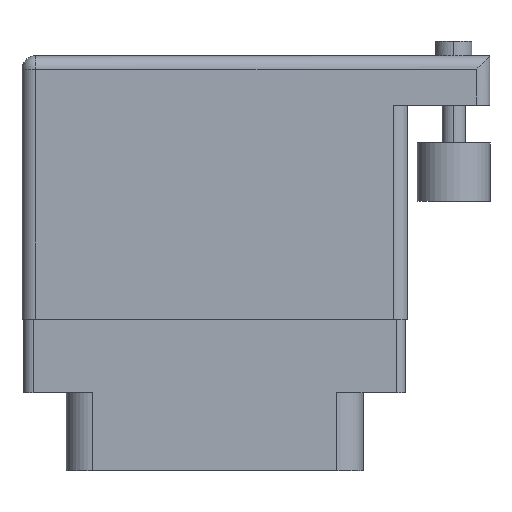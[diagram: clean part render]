
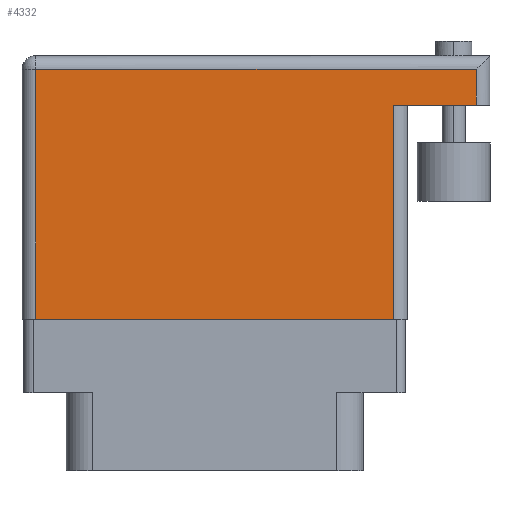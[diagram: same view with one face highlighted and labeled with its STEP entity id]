
A CAD part, front view. The second image highlights one B-rep face of the part: STEP entity #4332.
In plain terms, the highlighted face is planar.
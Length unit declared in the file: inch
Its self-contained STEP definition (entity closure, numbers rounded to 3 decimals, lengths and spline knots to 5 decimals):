
#379 = EDGE_CURVE ( 'NONE', #4389, #19625, #25853, .T. ) ;
#608 = EDGE_CURVE ( 'NONE', #2554, #6173, #16912, .T. ) ;
#660 = VECTOR ( 'NONE', #26076, 39.37008 ) ;
#966 = CARTESIAN_POINT ( 'NONE',  ( 1.278, 0.736, 0. ) ) ;
#1484 = VECTOR ( 'NONE', #26105, 39.37008 ) ;
#1532 = EDGE_LOOP ( 'NONE', ( #11667, #21692, #9767, #13888, #3674, #26341 ) ) ;
#2554 = VERTEX_POINT ( 'NONE', #25929 ) ;
#2714 = FACE_OUTER_BOUND ( 'NONE', #1532, .T. ) ;
#3550 = VERTEX_POINT ( 'NONE', #9226 ) ;
#3674 = ORIENTED_EDGE ( 'NONE', *, *, #4164, .T. ) ;
#3923 = DIRECTION ( 'NONE',  ( -1., 0., 0. ) ) ;
#4164 = EDGE_CURVE ( 'NONE', #6173, #3550, #26039, .T. ) ;
#4332 = ADVANCED_FACE ( 'NONE', ( #2714 ), #6448, .F. ) ;
#4389 = VERTEX_POINT ( 'NONE', #18974 ) ;
#4541 = CARTESIAN_POINT ( 'NONE',  ( 1.562, 0.859, 0. ) ) ;
#6173 = VERTEX_POINT ( 'NONE', #4541 ) ;
#6448 = PLANE ( 'NONE',  #23777 ) ;
#6714 = CARTESIAN_POINT ( 'NONE',  ( 0., 0.906, 0. ) ) ;
#6753 = LINE ( 'NONE', #9155, #11820 ) ;
#6914 = EDGE_CURVE ( 'NONE', #3550, #4389, #26202, .T. ) ;
#7649 = VERTEX_POINT ( 'NONE', #966 ) ;
#7923 = CARTESIAN_POINT ( 'NONE',  ( 0., 0.859, 0. ) ) ;
#9048 = CARTESIAN_POINT ( 'NONE',  ( 1.562, 0.906, 0. ) ) ;
#9155 = CARTESIAN_POINT ( 'NONE',  ( 1.278, 0.736, 0. ) ) ;
#9226 = CARTESIAN_POINT ( 'NONE',  ( 0.047, 0.859, 0. ) ) ;
#9767 = ORIENTED_EDGE ( 'NONE', *, *, #12261, .F. ) ;
#11430 = VECTOR ( 'NONE', #3923, 39.37008 ) ;
#11667 = ORIENTED_EDGE ( 'NONE', *, *, #379, .T. ) ;
#11820 = VECTOR ( 'NONE', #16752, 39.37008 ) ;
#12261 = EDGE_CURVE ( 'NONE', #2554, #7649, #13103, .T. ) ;
#12764 = VECTOR ( 'NONE', #19320, 39.37008 ) ;
#12830 = DIRECTION ( 'NONE',  ( -1., 0., 0. ) ) ;
#13103 = LINE ( 'NONE', #19375, #13503 ) ;
#13503 = VECTOR ( 'NONE', #24946, 39.37008 ) ;
#13888 = ORIENTED_EDGE ( 'NONE', *, *, #608, .T. ) ;
#13991 = CARTESIAN_POINT ( 'NONE',  ( 0., 0., 0. ) ) ;
#16161 = CARTESIAN_POINT ( 'NONE',  ( 1.278, 0., 0. ) ) ;
#16752 = DIRECTION ( 'NONE',  ( 0., 1., 0. ) ) ;
#16912 = LINE ( 'NONE', #9048, #12764 ) ;
#18974 = CARTESIAN_POINT ( 'NONE',  ( 0.047, 0., 0. ) ) ;
#19320 = DIRECTION ( 'NONE',  ( 0., 1., 0. ) ) ;
#19338 = EDGE_CURVE ( 'NONE', #19625, #7649, #6753, .T. ) ;
#19375 = CARTESIAN_POINT ( 'NONE',  ( 1.609, 0.736, 0. ) ) ;
#19625 = VERTEX_POINT ( 'NONE', #16161 ) ;
#20214 = CARTESIAN_POINT ( 'NONE',  ( 0.047, 0., 0. ) ) ;
#21692 = ORIENTED_EDGE ( 'NONE', *, *, #19338, .T. ) ;
#23777 = AXIS2_PLACEMENT_3D ( 'NONE', #6714, #24950, #12830 ) ;
#24946 = DIRECTION ( 'NONE',  ( -1., 0., 0. ) ) ;
#24950 = DIRECTION ( 'NONE',  ( 0., 0., -1. ) ) ;
#25853 = LINE ( 'NONE', #13991, #1484 ) ;
#25929 = CARTESIAN_POINT ( 'NONE',  ( 1.562, 0.736, 0. ) ) ;
#26039 = LINE ( 'NONE', #7923, #11430 ) ;
#26076 = DIRECTION ( 'NONE',  ( 0., -1., 0. ) ) ;
#26105 = DIRECTION ( 'NONE',  ( 1., 0., 0. ) ) ;
#26202 = LINE ( 'NONE', #20214, #660 ) ;
#26341 = ORIENTED_EDGE ( 'NONE', *, *, #6914, .T. ) ;
